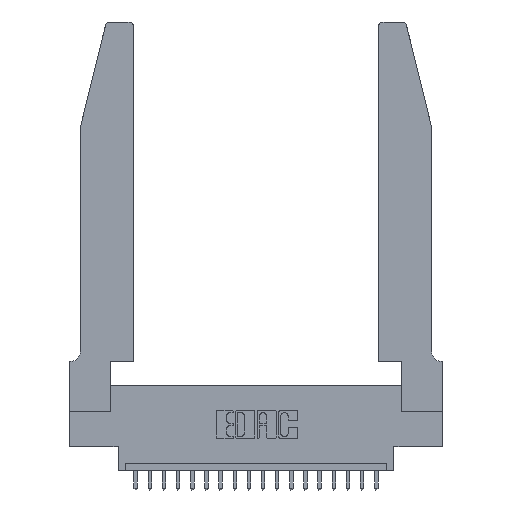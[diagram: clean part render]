
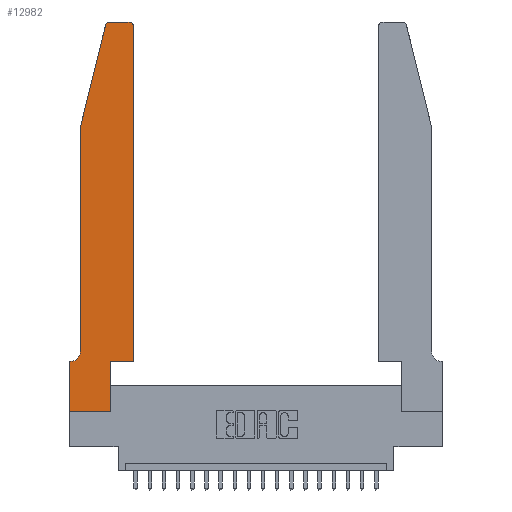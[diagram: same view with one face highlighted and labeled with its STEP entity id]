
A CAD part, top view. The second image highlights one B-rep face of the part: STEP entity #12982.
In plain terms, the highlighted planar face has unit normal (0, 0, 1).
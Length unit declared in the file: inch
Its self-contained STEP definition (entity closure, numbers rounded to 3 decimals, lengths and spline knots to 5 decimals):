
#237 = LINE ( 'NONE', #16848, #10691 ) ;
#259 = ORIENTED_EDGE ( 'NONE', *, *, #18346, .T. ) ;
#300 = CARTESIAN_POINT ( 'NONE',  ( 0.2605, 2.75, 0.37 ) ) ;
#567 = EDGE_CURVE ( 'NONE', #14343, #9480, #1012, .T. ) ;
#591 = VERTEX_POINT ( 'NONE', #18330 ) ;
#855 = EDGE_CURVE ( 'NONE', #591, #5878, #3895, .T. ) ;
#909 = VERTEX_POINT ( 'NONE', #9342 ) ;
#1012 = LINE ( 'NONE', #11621, #14668 ) ;
#1192 = EDGE_CURVE ( 'NONE', #5619, #909, #14925, .T. ) ;
#1256 = VECTOR ( 'NONE', #2235, 39.37008 ) ;
#1342 = VERTEX_POINT ( 'NONE', #13939 ) ;
#1506 = CARTESIAN_POINT ( 'NONE',  ( 0.4205, 2.75, 0.37 ) ) ;
#1770 = CIRCLE ( 'NONE', #11795, 0.03 ) ;
#2235 = DIRECTION ( 'NONE',  ( -0.239, -0.971, 0. ) ) ;
#3118 = EDGE_CURVE ( 'NONE', #12168, #18024, #3548, .T. ) ;
#3300 = DIRECTION ( 'NONE',  ( 0., -1., 0. ) ) ;
#3548 = LINE ( 'NONE', #18189, #7214 ) ;
#3873 = VECTOR ( 'NONE', #21649, 39.37008 ) ;
#3895 = CIRCLE ( 'NONE', #5615, 0.03 ) ;
#4374 = CARTESIAN_POINT ( 'NONE',  ( 0.0755, 0.42, 0.37 ) ) ;
#4522 = CARTESIAN_POINT ( 'NONE',  ( 0.2865, 0.35, 0.37 ) ) ;
#4962 = CARTESIAN_POINT ( 'NONE',  ( 0., 0., 0.37 ) ) ;
#5615 = AXIS2_PLACEMENT_3D ( 'NONE', #6068, #7528, #19335 ) ;
#5619 = VERTEX_POINT ( 'NONE', #4522 ) ;
#5878 = VERTEX_POINT ( 'NONE', #14852 ) ;
#6048 = CARTESIAN_POINT ( 'NONE',  ( 0.0755, 0.35, 0.37 ) ) ;
#6068 = CARTESIAN_POINT ( 'NONE',  ( 0.284, 2.72, 0.37 ) ) ;
#6144 = DIRECTION ( 'NONE',  ( 1., 0., 0. ) ) ;
#6221 = CARTESIAN_POINT ( 'NONE',  ( 0.2865, 0.35, 0.37 ) ) ;
#6702 = EDGE_CURVE ( 'NONE', #18024, #1342, #15645, .T. ) ;
#7214 = VECTOR ( 'NONE', #10037, 39.37008 ) ;
#7386 = VECTOR ( 'NONE', #11122, 39.37008 ) ;
#7528 = DIRECTION ( 'NONE',  ( 0., 0., 1. ) ) ;
#7670 = CIRCLE ( 'NONE', #19121, 0.07 ) ;
#7812 = VERTEX_POINT ( 'NONE', #21598 ) ;
#7935 = DIRECTION ( 'NONE',  ( 1., 0., 0. ) ) ;
#8087 = AXIS2_PLACEMENT_3D ( 'NONE', #16366, #9617, #7935 ) ;
#8104 = CARTESIAN_POINT ( 'NONE',  ( 0.4205, 2.72, 0.37 ) ) ;
#8338 = DIRECTION ( 'NONE',  ( 0., 1., 0. ) ) ;
#9007 = LINE ( 'NONE', #6048, #20577 ) ;
#9342 = CARTESIAN_POINT ( 'NONE',  ( 0.4505, 0.35, 0.37 ) ) ;
#9480 = VERTEX_POINT ( 'NONE', #4374 ) ;
#9617 = DIRECTION ( 'NONE',  ( 0., 0., 1. ) ) ;
#9632 = DIRECTION ( 'NONE',  ( 1., 0., 0. ) ) ;
#9690 = PLANE ( 'NONE',  #8087 ) ;
#10037 = DIRECTION ( 'NONE',  ( 0., -1., 0. ) ) ;
#10534 = VERTEX_POINT ( 'NONE', #17957 ) ;
#10691 = VECTOR ( 'NONE', #8338, 39.37008 ) ;
#11122 = DIRECTION ( 'NONE',  ( 0., 1., 0. ) ) ;
#11191 = VERTEX_POINT ( 'NONE', #1506 ) ;
#11207 = DIRECTION ( 'NONE',  ( -1., 0., 0. ) ) ;
#11621 = CARTESIAN_POINT ( 'NONE',  ( 0.0755, 2., 0.37 ) ) ;
#11795 = AXIS2_PLACEMENT_3D ( 'NONE', #8104, #18078, #6144 ) ;
#11817 = EDGE_CURVE ( 'NONE', #909, #7812, #237, .T. ) ;
#11941 = ORIENTED_EDGE ( 'NONE', *, *, #6702, .T. ) ;
#12168 = VERTEX_POINT ( 'NONE', #17519 ) ;
#12332 = ORIENTED_EDGE ( 'NONE', *, *, #19484, .T. ) ;
#12982 = ADVANCED_FACE ( 'NONE', ( #15518 ), #9690, .T. ) ;
#13655 = EDGE_LOOP ( 'NONE', ( #14808, #20351, #18605, #17997, #259, #20110, #16395, #11941, #18352, #14879, #14462, #12332 ) ) ;
#13850 = DIRECTION ( 'NONE',  ( -1., 0., 0. ) ) ;
#13939 = CARTESIAN_POINT ( 'NONE',  ( 0.2865, 0., 0.37 ) ) ;
#14132 = CARTESIAN_POINT ( 'NONE',  ( 0.0755, 2., 0.37 ) ) ;
#14343 = VERTEX_POINT ( 'NONE', #20270 ) ;
#14345 = DIRECTION ( 'NONE',  ( -1., 0., 0. ) ) ;
#14462 = ORIENTED_EDGE ( 'NONE', *, *, #11817, .T. ) ;
#14668 = VECTOR ( 'NONE', #3300, 39.37008 ) ;
#14780 = EDGE_CURVE ( 'NONE', #5878, #14343, #14885, .T. ) ;
#14808 = ORIENTED_EDGE ( 'NONE', *, *, #20226, .T. ) ;
#14852 = CARTESIAN_POINT ( 'NONE',  ( 0.25487, 2.72718, 0.37 ) ) ;
#14879 = ORIENTED_EDGE ( 'NONE', *, *, #1192, .T. ) ;
#14885 = LINE ( 'NONE', #14132, #1256 ) ;
#14925 = LINE ( 'NONE', #20253, #3873 ) ;
#15518 = FACE_OUTER_BOUND ( 'NONE', #13655, .T. ) ;
#15636 = LINE ( 'NONE', #300, #17740 ) ;
#15645 = LINE ( 'NONE', #18232, #20854 ) ;
#16075 = CARTESIAN_POINT ( 'NONE',  ( 0.0055, 0.42, 0.37 ) ) ;
#16366 = CARTESIAN_POINT ( 'NONE',  ( 0., 0.35, 0.37 ) ) ;
#16395 = ORIENTED_EDGE ( 'NONE', *, *, #3118, .T. ) ;
#16663 = EDGE_CURVE ( 'NONE', #10534, #12168, #9007, .T. ) ;
#16848 = CARTESIAN_POINT ( 'NONE',  ( 0.4505, 0.35, 0.37 ) ) ;
#17519 = CARTESIAN_POINT ( 'NONE',  ( 0., 0.35, 0.37 ) ) ;
#17616 = LINE ( 'NONE', #6221, #7386 ) ;
#17740 = VECTOR ( 'NONE', #13850, 39.37008 ) ;
#17957 = CARTESIAN_POINT ( 'NONE',  ( 0.0055, 0.35, 0.37 ) ) ;
#17997 = ORIENTED_EDGE ( 'NONE', *, *, #567, .T. ) ;
#18024 = VERTEX_POINT ( 'NONE', #4962 ) ;
#18078 = DIRECTION ( 'NONE',  ( 0., 0., 1. ) ) ;
#18189 = CARTESIAN_POINT ( 'NONE',  ( 0., 0., 0.37 ) ) ;
#18232 = CARTESIAN_POINT ( 'NONE',  ( 0., 0., 0.37 ) ) ;
#18330 = CARTESIAN_POINT ( 'NONE',  ( 0.284, 2.75, 0.37 ) ) ;
#18346 = EDGE_CURVE ( 'NONE', #9480, #10534, #7670, .T. ) ;
#18352 = ORIENTED_EDGE ( 'NONE', *, *, #19097, .T. ) ;
#18605 = ORIENTED_EDGE ( 'NONE', *, *, #14780, .T. ) ;
#19097 = EDGE_CURVE ( 'NONE', #1342, #5619, #17616, .T. ) ;
#19121 = AXIS2_PLACEMENT_3D ( 'NONE', #16075, #21259, #11207 ) ;
#19335 = DIRECTION ( 'NONE',  ( 1., 0., 0. ) ) ;
#19484 = EDGE_CURVE ( 'NONE', #7812, #11191, #1770, .T. ) ;
#20110 = ORIENTED_EDGE ( 'NONE', *, *, #16663, .T. ) ;
#20226 = EDGE_CURVE ( 'NONE', #11191, #591, #15636, .T. ) ;
#20253 = CARTESIAN_POINT ( 'NONE',  ( 0.4505, 0.35, 0.37 ) ) ;
#20270 = CARTESIAN_POINT ( 'NONE',  ( 0.0755, 2., 0.37 ) ) ;
#20351 = ORIENTED_EDGE ( 'NONE', *, *, #855, .T. ) ;
#20577 = VECTOR ( 'NONE', #14345, 39.37008 ) ;
#20854 = VECTOR ( 'NONE', #9632, 39.37008 ) ;
#21259 = DIRECTION ( 'NONE',  ( 0., 0., -1. ) ) ;
#21598 = CARTESIAN_POINT ( 'NONE',  ( 0.4505, 2.72, 0.37 ) ) ;
#21649 = DIRECTION ( 'NONE',  ( 1., 0., 0. ) ) ;
